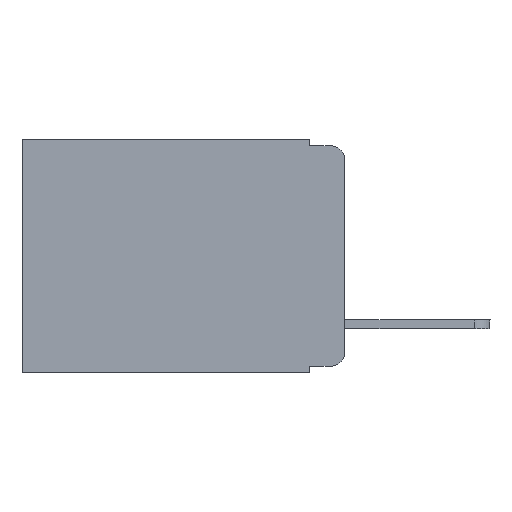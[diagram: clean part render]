
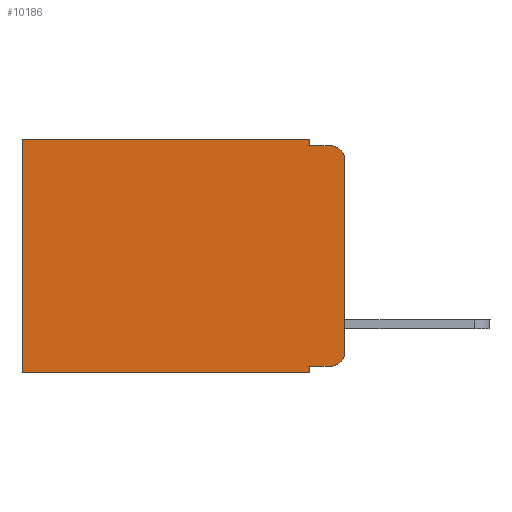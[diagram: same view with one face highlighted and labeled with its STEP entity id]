
A CAD part, left-side view. The second image highlights one B-rep face of the part: STEP entity #10186.
In plain terms, the highlighted planar face has unit normal (-1, 0, 0).
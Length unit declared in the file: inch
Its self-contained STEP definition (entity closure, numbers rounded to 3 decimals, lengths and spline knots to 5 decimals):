
#4 = EDGE_CURVE ( 'NONE', #8665, #9538, #2380, .T. ) ;
#174 = CARTESIAN_POINT ( 'NONE',  ( 0.298, 0.473, 0. ) ) ;
#295 = EDGE_CURVE ( 'NONE', #10136, #3964, #5987, .T. ) ;
#396 = ORIENTED_EDGE ( 'NONE', *, *, #5844, .T. ) ;
#638 = CARTESIAN_POINT ( 'NONE',  ( 0.298, 0.051, -0.343 ) ) ;
#751 = ORIENTED_EDGE ( 'NONE', *, *, #1152, .F. ) ;
#812 = EDGE_CURVE ( 'NONE', #8665, #7155, #4417, .T. ) ;
#1019 = VECTOR ( 'NONE', #10413, 39.37008 ) ;
#1055 = EDGE_LOOP ( 'NONE', ( #9588, #4075, #751, #9375, #2013, #396, #5754, #3986, #5607, #10191 ) ) ;
#1152 = EDGE_CURVE ( 'NONE', #4163, #3964, #7889, .T. ) ;
#1175 = DIRECTION ( 'NONE',  ( -1., 0., 0. ) ) ;
#1193 = VERTEX_POINT ( 'NONE', #2090 ) ;
#1876 = LINE ( 'NONE', #7971, #8350 ) ;
#1879 = CARTESIAN_POINT ( 'NONE',  ( 0.298, 0., 0. ) ) ;
#2010 = DIRECTION ( 'NONE',  ( 0., 0., -1. ) ) ;
#2013 = ORIENTED_EDGE ( 'NONE', *, *, #3363, .T. ) ;
#2090 = CARTESIAN_POINT ( 'NONE',  ( 0.298, 0.473, -0.343 ) ) ;
#2128 = CARTESIAN_POINT ( 'NONE',  ( 0.298, 0.02, -0.313 ) ) ;
#2380 = LINE ( 'NONE', #4637, #6542 ) ;
#2425 = AXIS2_PLACEMENT_3D ( 'NONE', #2128, #1175, #6987 ) ;
#2426 = CARTESIAN_POINT ( 'NONE',  ( 0.298, 0., 0. ) ) ;
#2552 = DIRECTION ( 'NONE',  ( -1., 0., 0. ) ) ;
#2561 = VERTEX_POINT ( 'NONE', #9532 ) ;
#2591 = EDGE_CURVE ( 'NONE', #10136, #2561, #4230, .T. ) ;
#2820 = AXIS2_PLACEMENT_3D ( 'NONE', #2426, #7997, #3031 ) ;
#3031 = DIRECTION ( 'NONE',  ( 0., 0., -1. ) ) ;
#3324 = LINE ( 'NONE', #7164, #7496 ) ;
#3363 = EDGE_CURVE ( 'NONE', #6320, #6374, #5378, .T. ) ;
#3479 = DIRECTION ( 'NONE',  ( 0., 1., 0. ) ) ;
#3778 = CARTESIAN_POINT ( 'NONE',  ( 0.298, 0.473, 0. ) ) ;
#3823 = DIRECTION ( 'NONE',  ( 0., 1., 0. ) ) ;
#3964 = VERTEX_POINT ( 'NONE', #9718 ) ;
#3986 = ORIENTED_EDGE ( 'NONE', *, *, #812, .F. ) ;
#4075 = ORIENTED_EDGE ( 'NONE', *, *, #295, .T. ) ;
#4163 = VERTEX_POINT ( 'NONE', #10385 ) ;
#4230 = LINE ( 'NONE', #4430, #7357 ) ;
#4417 = LINE ( 'NONE', #5789, #7423 ) ;
#4430 = CARTESIAN_POINT ( 'NONE',  ( 0.298, 0., 0. ) ) ;
#4637 = CARTESIAN_POINT ( 'NONE',  ( 0.298, 0.051, -0.333 ) ) ;
#5052 = EDGE_CURVE ( 'NONE', #6320, #4163, #1876, .T. ) ;
#5378 = LINE ( 'NONE', #1879, #7086 ) ;
#5545 = CARTESIAN_POINT ( 'NONE',  ( 0.298, 0.02, -0.333 ) ) ;
#5607 = ORIENTED_EDGE ( 'NONE', *, *, #4, .T. ) ;
#5754 = ORIENTED_EDGE ( 'NONE', *, *, #9548, .F. ) ;
#5786 = PLANE ( 'NONE',  #2820 ) ;
#5789 = CARTESIAN_POINT ( 'NONE',  ( 0.298, 0.051, 0. ) ) ;
#5830 = CARTESIAN_POINT ( 'NONE',  ( 0.298, 0.051, 0. ) ) ;
#5844 = EDGE_CURVE ( 'NONE', #6374, #1193, #6132, .T. ) ;
#5871 = VECTOR ( 'NONE', #2010, 39.37008 ) ;
#5987 = CIRCLE ( 'NONE', #7455, 0.02 ) ;
#6132 = LINE ( 'NONE', #3778, #5871 ) ;
#6160 = CARTESIAN_POINT ( 'NONE',  ( 0.298, 0., -0.03 ) ) ;
#6166 = DIRECTION ( 'NONE',  ( 0., 0., -1. ) ) ;
#6237 = DIRECTION ( 'NONE',  ( 0., -1., 0. ) ) ;
#6319 = CARTESIAN_POINT ( 'NONE',  ( 0.298, 0.051, -0.01 ) ) ;
#6320 = VERTEX_POINT ( 'NONE', #5830 ) ;
#6374 = VERTEX_POINT ( 'NONE', #174 ) ;
#6542 = VECTOR ( 'NONE', #6237, 39.37008 ) ;
#6660 = CARTESIAN_POINT ( 'NONE',  ( 0.298, 0.02, -0.03 ) ) ;
#6963 = DIRECTION ( 'NONE',  ( 0., 0., -1. ) ) ;
#6987 = DIRECTION ( 'NONE',  ( 0., 0., -1. ) ) ;
#7075 = EDGE_CURVE ( 'NONE', #9538, #2561, #8424, .T. ) ;
#7086 = VECTOR ( 'NONE', #3479, 39.37008 ) ;
#7155 = VERTEX_POINT ( 'NONE', #638 ) ;
#7164 = CARTESIAN_POINT ( 'NONE',  ( 0.298, 0., -0.343 ) ) ;
#7357 = VECTOR ( 'NONE', #6963, 39.37008 ) ;
#7370 = DIRECTION ( 'NONE',  ( 0., 0., -1. ) ) ;
#7423 = VECTOR ( 'NONE', #9318, 39.37008 ) ;
#7455 = AXIS2_PLACEMENT_3D ( 'NONE', #6660, #2552, #7370 ) ;
#7496 = VECTOR ( 'NONE', #3823, 39.37008 ) ;
#7889 = LINE ( 'NONE', #6319, #1019 ) ;
#7971 = CARTESIAN_POINT ( 'NONE',  ( 0.298, 0.051, 0. ) ) ;
#7997 = DIRECTION ( 'NONE',  ( 1., 0., 0. ) ) ;
#8350 = VECTOR ( 'NONE', #6166, 39.37008 ) ;
#8373 = FACE_OUTER_BOUND ( 'NONE', #1055, .T. ) ;
#8422 = CARTESIAN_POINT ( 'NONE',  ( 0.298, 0.051, -0.333 ) ) ;
#8424 = CIRCLE ( 'NONE', #2425, 0.02 ) ;
#8665 = VERTEX_POINT ( 'NONE', #8422 ) ;
#9318 = DIRECTION ( 'NONE',  ( 0., 0., -1. ) ) ;
#9375 = ORIENTED_EDGE ( 'NONE', *, *, #5052, .F. ) ;
#9532 = CARTESIAN_POINT ( 'NONE',  ( 0.298, 0., -0.313 ) ) ;
#9538 = VERTEX_POINT ( 'NONE', #5545 ) ;
#9548 = EDGE_CURVE ( 'NONE', #7155, #1193, #3324, .T. ) ;
#9588 = ORIENTED_EDGE ( 'NONE', *, *, #2591, .F. ) ;
#9718 = CARTESIAN_POINT ( 'NONE',  ( 0.298, 0.02, -0.01 ) ) ;
#10136 = VERTEX_POINT ( 'NONE', #6160 ) ;
#10186 = ADVANCED_FACE ( 'NONE', ( #8373 ), #5786, .F. ) ;
#10191 = ORIENTED_EDGE ( 'NONE', *, *, #7075, .T. ) ;
#10385 = CARTESIAN_POINT ( 'NONE',  ( 0.298, 0.051, -0.01 ) ) ;
#10413 = DIRECTION ( 'NONE',  ( 0., -1., 0. ) ) ;
